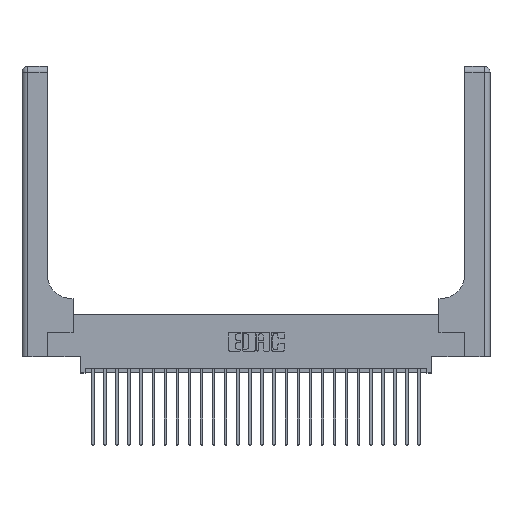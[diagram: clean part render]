
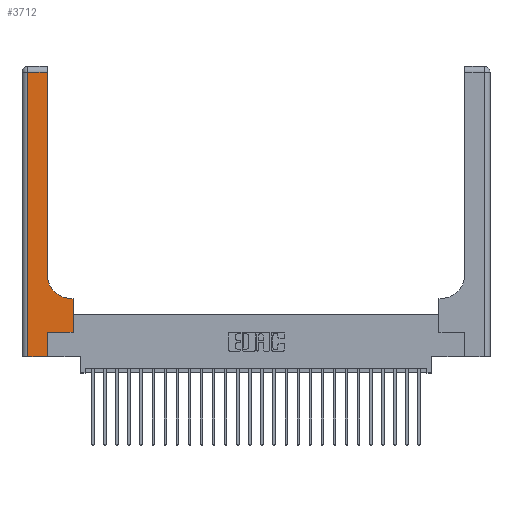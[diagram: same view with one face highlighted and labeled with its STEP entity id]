
A CAD part, top view. The second image highlights one B-rep face of the part: STEP entity #3712.
In plain terms, the highlighted planar face has unit normal (0, 0, 1).
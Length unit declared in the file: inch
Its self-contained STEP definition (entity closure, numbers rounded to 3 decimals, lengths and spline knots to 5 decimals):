
#434 = ORIENTED_EDGE ( 'NONE', *, *, #17057, .T. ) ;
#1058 = VERTEX_POINT ( 'NONE', #10715 ) ;
#1142 = CARTESIAN_POINT ( 'NONE',  ( 0.06, 3., 0.37 ) ) ;
#1242 = CARTESIAN_POINT ( 'NONE',  ( 0.26, 0.85, 0.37 ) ) ;
#1655 = VERTEX_POINT ( 'NONE', #1242 ) ;
#2574 = ORIENTED_EDGE ( 'NONE', *, *, #13145, .T. ) ;
#2912 = ORIENTED_EDGE ( 'NONE', *, *, #4738, .T. ) ;
#3357 = DIRECTION ( 'NONE',  ( 0., 1., 0. ) ) ;
#3712 = ADVANCED_FACE ( 'NONE', ( #10498 ), #4310, .F. ) ;
#3830 = VECTOR ( 'NONE', #17400, 39.37008 ) ;
#3963 = VECTOR ( 'NONE', #5111, 39.37008 ) ;
#4055 = CARTESIAN_POINT ( 'NONE',  ( 0., 3., 0.37 ) ) ;
#4310 = PLANE ( 'NONE',  #22054 ) ;
#4332 = VERTEX_POINT ( 'NONE', #22892 ) ;
#4738 = EDGE_CURVE ( 'NONE', #7274, #7090, #9078, .T. ) ;
#5111 = DIRECTION ( 'NONE',  ( 0., 1., 0. ) ) ;
#5120 = ORIENTED_EDGE ( 'NONE', *, *, #6844, .T. ) ;
#5327 = EDGE_CURVE ( 'NONE', #7090, #4332, #5489, .T. ) ;
#5489 = LINE ( 'NONE', #11392, #10112 ) ;
#5874 = VERTEX_POINT ( 'NONE', #10534 ) ;
#6089 = AXIS2_PLACEMENT_3D ( 'NONE', #7837, #15823, #20152 ) ;
#6571 = DIRECTION ( 'NONE',  ( 0., 0., -1. ) ) ;
#6844 = EDGE_CURVE ( 'NONE', #4332, #1058, #10336, .T. ) ;
#6897 = VECTOR ( 'NONE', #17675, 39.37008 ) ;
#7090 = VERTEX_POINT ( 'NONE', #15131 ) ;
#7274 = VERTEX_POINT ( 'NONE', #8032 ) ;
#7837 = CARTESIAN_POINT ( 'NONE',  ( 0.51, 0.85, 0.37 ) ) ;
#8032 = CARTESIAN_POINT ( 'NONE',  ( 0.06, 0., 0.37 ) ) ;
#8447 = CARTESIAN_POINT ( 'NONE',  ( 0.26, 2.94, 0.37 ) ) ;
#9078 = LINE ( 'NONE', #17087, #19895 ) ;
#9704 = EDGE_CURVE ( 'NONE', #1058, #5874, #11358, .T. ) ;
#9731 = VECTOR ( 'NONE', #10310, 39.37008 ) ;
#9898 = ORIENTED_EDGE ( 'NONE', *, *, #9704, .T. ) ;
#10112 = VECTOR ( 'NONE', #17694, 39.37008 ) ;
#10310 = DIRECTION ( 'NONE',  ( -1., 0., 0. ) ) ;
#10336 = LINE ( 'NONE', #23988, #21010 ) ;
#10498 = FACE_OUTER_BOUND ( 'NONE', #15218, .T. ) ;
#10523 = CARTESIAN_POINT ( 'NONE',  ( 0.51, 0.6, 0.37 ) ) ;
#10534 = CARTESIAN_POINT ( 'NONE',  ( 0.528, 0.6, 0.37 ) ) ;
#10715 = CARTESIAN_POINT ( 'NONE',  ( 0.528, 0.25, 0.37 ) ) ;
#11358 = LINE ( 'NONE', #21333, #17820 ) ;
#11392 = CARTESIAN_POINT ( 'NONE',  ( 0.265, 0., 0.37 ) ) ;
#11750 = LINE ( 'NONE', #1142, #3830 ) ;
#13002 = EDGE_CURVE ( 'NONE', #24667, #7274, #11750, .T. ) ;
#13145 = EDGE_CURVE ( 'NONE', #18300, #1655, #17396, .T. ) ;
#13590 = CARTESIAN_POINT ( 'NONE',  ( 0.26, 0.6, 0.37 ) ) ;
#14282 = DIRECTION ( 'NONE',  ( -1., 0., 0. ) ) ;
#14357 = LINE ( 'NONE', #22257, #9731 ) ;
#14376 = EDGE_CURVE ( 'NONE', #24499, #24667, #14357, .T. ) ;
#15131 = CARTESIAN_POINT ( 'NONE',  ( 0.265, 0., 0.37 ) ) ;
#15218 = EDGE_LOOP ( 'NONE', ( #22985, #18384, #25188, #2912, #18478, #5120, #9898, #434, #2574 ) ) ;
#15823 = DIRECTION ( 'NONE',  ( 0., 0., -1. ) ) ;
#16492 = DIRECTION ( 'NONE',  ( 1., 0., 0. ) ) ;
#16663 = CARTESIAN_POINT ( 'NONE',  ( 0.26, 3., 0.37 ) ) ;
#17057 = EDGE_CURVE ( 'NONE', #5874, #18300, #21750, .T. ) ;
#17087 = CARTESIAN_POINT ( 'NONE',  ( 0., 0., 0.37 ) ) ;
#17396 = CIRCLE ( 'NONE', #6089, 0.25 ) ;
#17400 = DIRECTION ( 'NONE',  ( 0., -1., 0. ) ) ;
#17675 = DIRECTION ( 'NONE',  ( -1., 0., 0. ) ) ;
#17694 = DIRECTION ( 'NONE',  ( 0., 1., 0. ) ) ;
#17820 = VECTOR ( 'NONE', #3357, 39.37008 ) ;
#18300 = VERTEX_POINT ( 'NONE', #10523 ) ;
#18384 = ORIENTED_EDGE ( 'NONE', *, *, #14376, .T. ) ;
#18478 = ORIENTED_EDGE ( 'NONE', *, *, #5327, .T. ) ;
#19183 = CARTESIAN_POINT ( 'NONE',  ( 0.06, 2.94, 0.37 ) ) ;
#19895 = VECTOR ( 'NONE', #25098, 39.37008 ) ;
#19968 = EDGE_CURVE ( 'NONE', #1655, #24499, #20997, .T. ) ;
#20152 = DIRECTION ( 'NONE',  ( 1., 0., 0. ) ) ;
#20997 = LINE ( 'NONE', #16663, #3963 ) ;
#21010 = VECTOR ( 'NONE', #16492, 39.37008 ) ;
#21333 = CARTESIAN_POINT ( 'NONE',  ( 0.528, 0.25, 0.37 ) ) ;
#21750 = LINE ( 'NONE', #13590, #6897 ) ;
#22054 = AXIS2_PLACEMENT_3D ( 'NONE', #4055, #6571, #14282 ) ;
#22257 = CARTESIAN_POINT ( 'NONE',  ( 0., 2.94, 0.37 ) ) ;
#22892 = CARTESIAN_POINT ( 'NONE',  ( 0.265, 0.25, 0.37 ) ) ;
#22985 = ORIENTED_EDGE ( 'NONE', *, *, #19968, .T. ) ;
#23988 = CARTESIAN_POINT ( 'NONE',  ( 0.265, 0.25, 0.37 ) ) ;
#24499 = VERTEX_POINT ( 'NONE', #8447 ) ;
#24667 = VERTEX_POINT ( 'NONE', #19183 ) ;
#25098 = DIRECTION ( 'NONE',  ( 1., 0., 0. ) ) ;
#25188 = ORIENTED_EDGE ( 'NONE', *, *, #13002, .T. ) ;
